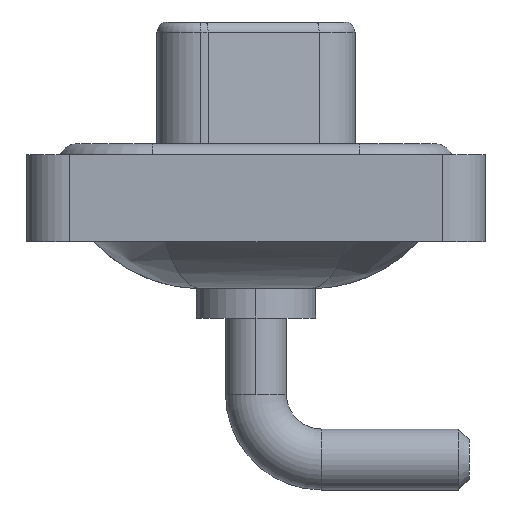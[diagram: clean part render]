
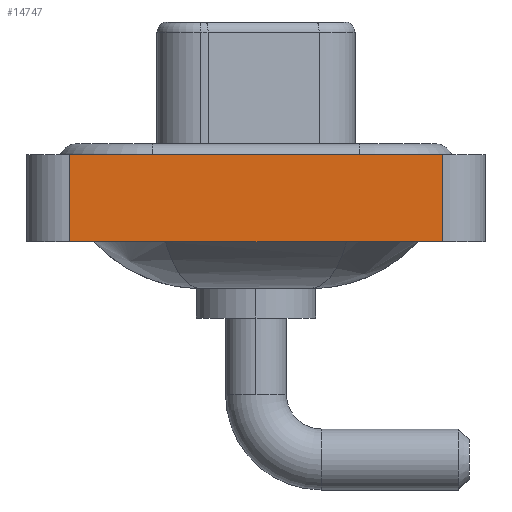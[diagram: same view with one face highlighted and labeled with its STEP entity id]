
A CAD part, left-side view. The second image highlights one B-rep face of the part: STEP entity #14747.
In plain terms, the highlighted planar face has unit normal (-1, 0, 0).
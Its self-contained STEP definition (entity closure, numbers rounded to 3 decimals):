
#133 = CARTESIAN_POINT ( 'NONE',  ( -7.3, -8.55, -3.6 ) ) ;
#474 = LINE ( 'NONE', #2788, #10260 ) ;
#476 = VERTEX_POINT ( 'NONE', #133 ) ;
#824 = PLANE ( 'NONE',  #9472 ) ;
#1703 = DIRECTION ( 'NONE',  ( 0., 0., 1. ) ) ;
#2669 = CARTESIAN_POINT ( 'NONE',  ( -7.3, -8.55, -3.6 ) ) ;
#2788 = CARTESIAN_POINT ( 'NONE',  ( -7.3, -8.55, -3.6 ) ) ;
#2981 = LINE ( 'NONE', #2669, #3927 ) ;
#3663 = VERTEX_POINT ( 'NONE', #15960 ) ;
#3909 = DIRECTION ( 'NONE',  ( 0., 0., 1. ) ) ;
#3927 = VECTOR ( 'NONE', #6661, 1000. ) ;
#4105 = EDGE_LOOP ( 'NONE', ( #5491, #10944, #4314, #12996 ) ) ;
#4314 = ORIENTED_EDGE ( 'NONE', *, *, #11958, .F. ) ;
#4382 = CARTESIAN_POINT ( 'NONE',  ( -7.3, -8.55, 0.4 ) ) ;
#4618 = DIRECTION ( 'NONE',  ( 0., -1., 0. ) ) ;
#4645 = DIRECTION ( 'NONE',  ( -1., 0., 0. ) ) ;
#4718 = LINE ( 'NONE', #4382, #11851 ) ;
#5491 = ORIENTED_EDGE ( 'NONE', *, *, #14111, .T. ) ;
#5545 = CARTESIAN_POINT ( 'NONE',  ( -7.3, 8.55, -3.6 ) ) ;
#5899 = CARTESIAN_POINT ( 'NONE',  ( -7.3, -8.55, -3.6 ) ) ;
#6661 = DIRECTION ( 'NONE',  ( 0., -1., 0. ) ) ;
#7654 = VERTEX_POINT ( 'NONE', #5545 ) ;
#7776 = CARTESIAN_POINT ( 'NONE',  ( -7.3, 8.55, -3.6 ) ) ;
#9048 = LINE ( 'NONE', #7776, #14052 ) ;
#9472 = AXIS2_PLACEMENT_3D ( 'NONE', #5899, #4645, #3909 ) ;
#10260 = VECTOR ( 'NONE', #1703, 1000. ) ;
#10944 = ORIENTED_EDGE ( 'NONE', *, *, #13848, .F. ) ;
#11473 = DIRECTION ( 'NONE',  ( 0., 0., 1. ) ) ;
#11722 = EDGE_CURVE ( 'NONE', #7654, #476, #2981, .T. ) ;
#11851 = VECTOR ( 'NONE', #4618, 1000. ) ;
#11958 = EDGE_CURVE ( 'NONE', #7654, #3663, #9048, .T. ) ;
#12244 = FACE_OUTER_BOUND ( 'NONE', #4105, .T. ) ;
#12996 = ORIENTED_EDGE ( 'NONE', *, *, #11722, .T. ) ;
#13848 = EDGE_CURVE ( 'NONE', #3663, #15758, #4718, .T. ) ;
#14052 = VECTOR ( 'NONE', #11473, 1000. ) ;
#14111 = EDGE_CURVE ( 'NONE', #476, #15758, #474, .T. ) ;
#14119 = CARTESIAN_POINT ( 'NONE',  ( -7.3, -8.55, 0.4 ) ) ;
#14747 = ADVANCED_FACE ( 'NONE', ( #12244 ), #824, .T. ) ;
#15758 = VERTEX_POINT ( 'NONE', #14119 ) ;
#15960 = CARTESIAN_POINT ( 'NONE',  ( -7.3, 8.55, 0.4 ) ) ;
